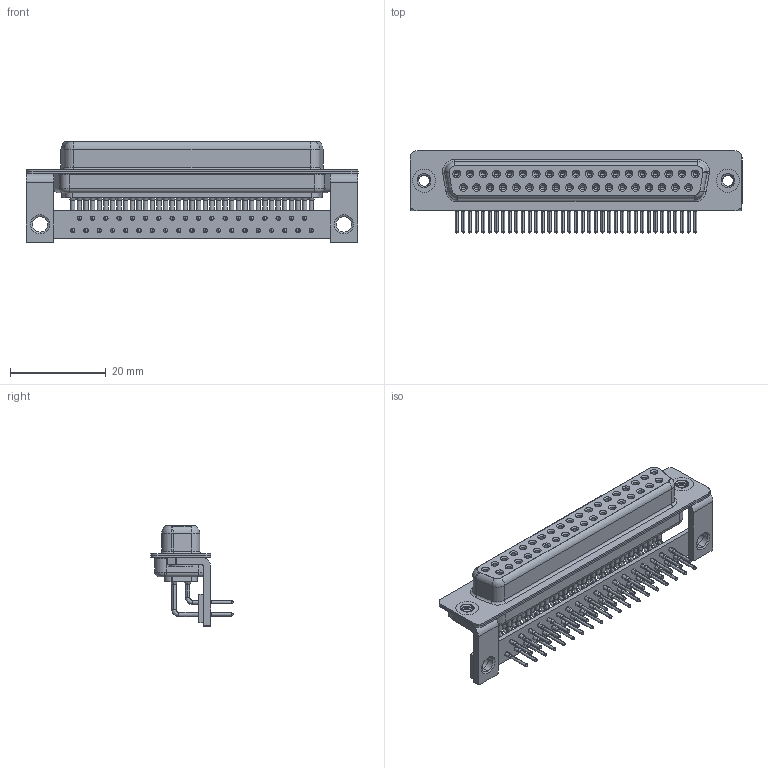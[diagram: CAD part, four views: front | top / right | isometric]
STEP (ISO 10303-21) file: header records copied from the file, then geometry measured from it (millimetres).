
FILE_DESCRIPTION (( 'STEP AP203' ), '1' );
FILE_NAME ('630-M37-340-GT4.STEP', '2018-09-26T05:32:46', ( '' ), ( '' ), 'SwSTEP 2.0', 'SolidWorks 2016', '' );
FILE_SCHEMA (( 'CONFIG_CONTROL_DESIGN' ));
Length unit declared in the file: millimetre
Products named in the file (9): 630M 4-40 Threaded Rivet_Stabilizer; 630M Stabilizer Bracket; 630M Stabilizer Board_37 Contacts; 630-M37-340-GT4; 630M Housing_37 Contacts; 630M Shell Front_37 Contacts; 630M Shell Rear_37 Contacts; 630M Contact Row 1; 630M Contact Row 2
Assembly tree (45 placements, depth 2):
  630-M37-340-GT4
    630M Housing_37 Contacts
    630M Shell Front_37 Contacts
    630M Shell Rear_37 Contacts
    630M Contact Row 1  x19
    630M Contact Row 2  x18
    630M 4-40 Threaded Rivet_Stabilizer  x2
    630M Stabilizer Bracket  x2
    630M Stabilizer Board_37 Contacts
Bounding box: 69.4 x 17.2 x 21 mm (x, y, z)
Volume: 6129.9 mm3; surface area: 15138.8 mm2
Topology: 45 solids, 45 shells, 2364 faces, 6034 edges, 3808 vertices
Faces by surface type: cylinder 1084, plane 648, cone 415, bspline 154, torus 63
Entity records: 30618 total; most frequent: CARTESIAN_POINT 6275, DIRECTION 5187, ORIENTED_EDGE 4292, AXIS2_PLACEMENT_3D 2182, EDGE_CURVE 2146, VERTEX_POINT 1375, CIRCLE 1234, EDGE_LOOP 1205
